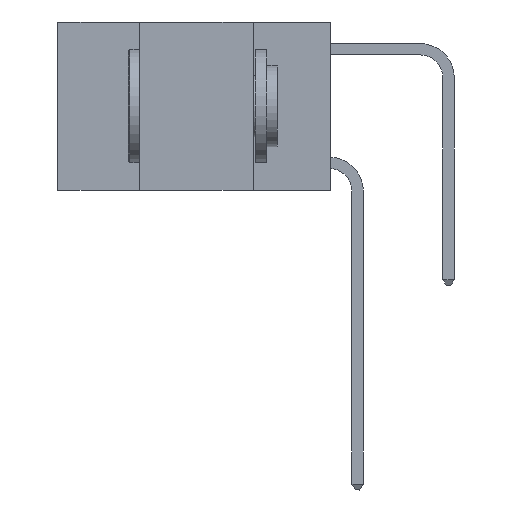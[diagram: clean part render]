
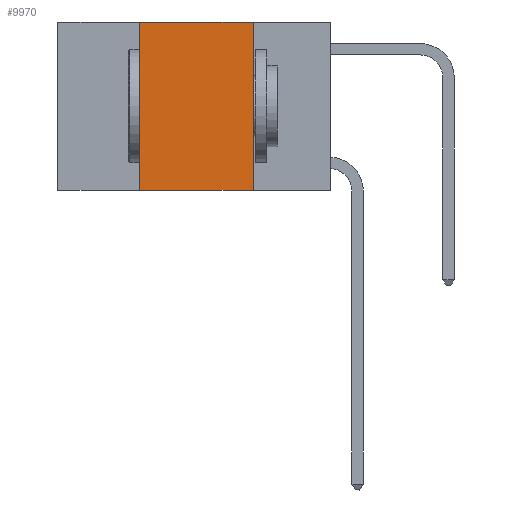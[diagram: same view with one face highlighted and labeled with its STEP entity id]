
A CAD part, left-side view. The second image highlights one B-rep face of the part: STEP entity #9970.
In plain terms, the highlighted planar face has unit normal (-1, 0, 0).
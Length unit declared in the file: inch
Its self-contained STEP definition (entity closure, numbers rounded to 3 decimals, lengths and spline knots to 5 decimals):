
#744 = CARTESIAN_POINT ( 'NONE',  ( 0., 0.42, 0. ) ) ;
#1631 = VERTEX_POINT ( 'NONE', #13800 ) ;
#1853 = EDGE_CURVE ( 'NONE', #2017, #6287, #9292, .T. ) ;
#2017 = VERTEX_POINT ( 'NONE', #14787 ) ;
#4200 = PLANE ( 'NONE',  #12021 ) ;
#5048 = EDGE_CURVE ( 'NONE', #2017, #11482, #10512, .T. ) ;
#5247 = ORIENTED_EDGE ( 'NONE', *, *, #5048, .T. ) ;
#5395 = LINE ( 'NONE', #9407, #13341 ) ;
#5529 = FACE_OUTER_BOUND ( 'NONE', #13086, .T. ) ;
#5787 = DIRECTION ( 'NONE',  ( 0., 0., 1. ) ) ;
#6287 = VERTEX_POINT ( 'NONE', #11099 ) ;
#8157 = DIRECTION ( 'NONE',  ( 0., -1., 0. ) ) ;
#9054 = EDGE_CURVE ( 'NONE', #6287, #1631, #5395, .T. ) ;
#9292 = LINE ( 'NONE', #744, #14524 ) ;
#9365 = DIRECTION ( 'NONE',  ( 1., 0., 0. ) ) ;
#9407 = CARTESIAN_POINT ( 'NONE',  ( 0., 0.6, 0. ) ) ;
#9803 = CARTESIAN_POINT ( 'NONE',  ( 0., 0.17, 0. ) ) ;
#9880 = DIRECTION ( 'NONE',  ( 0., 0., -1. ) ) ;
#9970 = ADVANCED_FACE ( 'NONE', ( #5529 ), #4200, .F. ) ;
#10512 = LINE ( 'NONE', #11758, #13147 ) ;
#11042 = LINE ( 'NONE', #9803, #12640 ) ;
#11099 = CARTESIAN_POINT ( 'NONE',  ( 0., 0.42, 0. ) ) ;
#11482 = VERTEX_POINT ( 'NONE', #11918 ) ;
#11758 = CARTESIAN_POINT ( 'NONE',  ( 0., 0.6, -0.37 ) ) ;
#11869 = CARTESIAN_POINT ( 'NONE',  ( 0., 0.6, 0. ) ) ;
#11918 = CARTESIAN_POINT ( 'NONE',  ( 0., 0.17, -0.37 ) ) ;
#12021 = AXIS2_PLACEMENT_3D ( 'NONE', #11869, #9365, #14191 ) ;
#12640 = VECTOR ( 'NONE', #9880, 39.37008 ) ;
#13086 = EDGE_LOOP ( 'NONE', ( #15626, #14212, #14260, #5247 ) ) ;
#13147 = VECTOR ( 'NONE', #15587, 39.37008 ) ;
#13341 = VECTOR ( 'NONE', #8157, 39.37008 ) ;
#13800 = CARTESIAN_POINT ( 'NONE',  ( 0., 0.17, 0. ) ) ;
#14191 = DIRECTION ( 'NONE',  ( 0., 0., -1. ) ) ;
#14212 = ORIENTED_EDGE ( 'NONE', *, *, #9054, .F. ) ;
#14260 = ORIENTED_EDGE ( 'NONE', *, *, #1853, .F. ) ;
#14524 = VECTOR ( 'NONE', #5787, 39.37008 ) ;
#14787 = CARTESIAN_POINT ( 'NONE',  ( 0., 0.42, -0.37 ) ) ;
#14973 = EDGE_CURVE ( 'NONE', #1631, #11482, #11042, .T. ) ;
#15587 = DIRECTION ( 'NONE',  ( 0., -1., 0. ) ) ;
#15626 = ORIENTED_EDGE ( 'NONE', *, *, #14973, .F. ) ;
